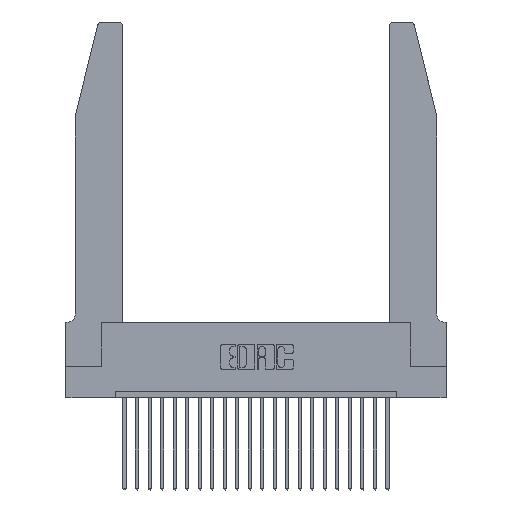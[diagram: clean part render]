
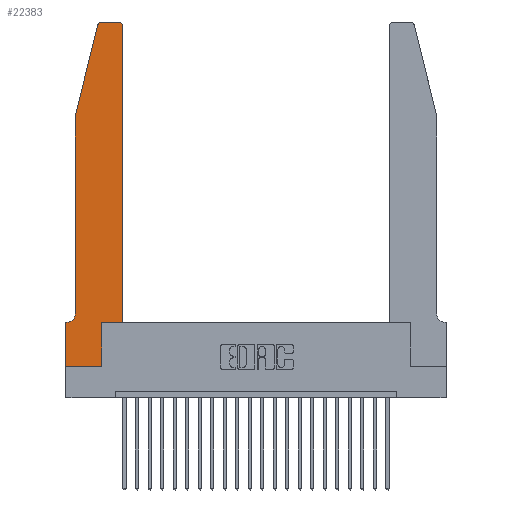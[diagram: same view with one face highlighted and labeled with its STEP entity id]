
A CAD part, top view. The second image highlights one B-rep face of the part: STEP entity #22383.
In plain terms, the highlighted planar face has unit normal (0, 0, 1).
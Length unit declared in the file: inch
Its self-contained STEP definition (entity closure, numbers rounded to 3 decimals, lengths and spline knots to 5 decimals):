
#57 = EDGE_CURVE ( 'NONE', #18648, #10782, #5771, .T. ) ;
#76 = DIRECTION ( 'NONE',  ( 0., 0., 1. ) ) ;
#520 = CARTESIAN_POINT ( 'NONE',  ( 0.0055, 0.35, 0.37 ) ) ;
#789 = VECTOR ( 'NONE', #22479, 39.37008 ) ;
#925 = VERTEX_POINT ( 'NONE', #14984 ) ;
#985 = CARTESIAN_POINT ( 'NONE',  ( 0., 0., 0.37 ) ) ;
#1343 = CARTESIAN_POINT ( 'NONE',  ( 0.25487, 2.72718, 0.37 ) ) ;
#1542 = DIRECTION ( 'NONE',  ( -1., 0., 0. ) ) ;
#2659 = VECTOR ( 'NONE', #9525, 39.37008 ) ;
#2760 = LINE ( 'NONE', #3527, #7111 ) ;
#2867 = VERTEX_POINT ( 'NONE', #16694 ) ;
#2967 = ORIENTED_EDGE ( 'NONE', *, *, #15690, .T. ) ;
#3189 = DIRECTION ( 'NONE',  ( 0., 0., 1. ) ) ;
#3259 = VECTOR ( 'NONE', #15316, 39.37008 ) ;
#3527 = CARTESIAN_POINT ( 'NONE',  ( 0.0755, 0.35, 0.37 ) ) ;
#3713 = VERTEX_POINT ( 'NONE', #18290 ) ;
#3759 = DIRECTION ( 'NONE',  ( -0.239, -0.971, 0. ) ) ;
#4540 = LINE ( 'NONE', #6917, #12961 ) ;
#4722 = CIRCLE ( 'NONE', #13330, 0.03 ) ;
#5266 = EDGE_CURVE ( 'NONE', #13035, #9064, #4540, .T. ) ;
#5589 = ORIENTED_EDGE ( 'NONE', *, *, #16961, .T. ) ;
#5689 = CARTESIAN_POINT ( 'NONE',  ( 0.0755, 2., 0.37 ) ) ;
#5757 = EDGE_CURVE ( 'NONE', #21542, #925, #2760, .T. ) ;
#5771 = LINE ( 'NONE', #13590, #789 ) ;
#6016 = VECTOR ( 'NONE', #3759, 39.37008 ) ;
#6346 = DIRECTION ( 'NONE',  ( 0., -1., 0. ) ) ;
#6392 = DIRECTION ( 'NONE',  ( 1., 0., 0. ) ) ;
#6635 = AXIS2_PLACEMENT_3D ( 'NONE', #16191, #10745, #7147 ) ;
#6715 = LINE ( 'NONE', #20277, #12856 ) ;
#6917 = CARTESIAN_POINT ( 'NONE',  ( 0.2605, 2.75, 0.37 ) ) ;
#6986 = EDGE_CURVE ( 'NONE', #9064, #9731, #4722, .T. ) ;
#7058 = EDGE_CURVE ( 'NONE', #19917, #3713, #15735, .T. ) ;
#7111 = VECTOR ( 'NONE', #1542, 39.37008 ) ;
#7147 = DIRECTION ( 'NONE',  ( -1., 0., 0. ) ) ;
#7605 = CARTESIAN_POINT ( 'NONE',  ( 0.2865, 0.35, 0.37 ) ) ;
#8390 = EDGE_LOOP ( 'NONE', ( #17396, #19748, #16897, #23469, #23577, #16543, #2967, #21806, #5589, #14961, #10084, #13837 ) ) ;
#8466 = CARTESIAN_POINT ( 'NONE',  ( 0., 0., 0.37 ) ) ;
#8567 = CIRCLE ( 'NONE', #9382, 0.03 ) ;
#8801 = DIRECTION ( 'NONE',  ( -1., 0., 0. ) ) ;
#9064 = VERTEX_POINT ( 'NONE', #21634 ) ;
#9091 = DIRECTION ( 'NONE',  ( 1., 0., 0. ) ) ;
#9142 = VECTOR ( 'NONE', #6346, 39.37008 ) ;
#9382 = AXIS2_PLACEMENT_3D ( 'NONE', #16250, #3189, #16169 ) ;
#9525 = DIRECTION ( 'NONE',  ( 0., -1., 0. ) ) ;
#9731 = VERTEX_POINT ( 'NONE', #1343 ) ;
#9945 = CARTESIAN_POINT ( 'NONE',  ( 0.4205, 2.75, 0.37 ) ) ;
#10084 = ORIENTED_EDGE ( 'NONE', *, *, #18473, .T. ) ;
#10219 = CARTESIAN_POINT ( 'NONE',  ( 0.4505, 0.35, 0.37 ) ) ;
#10232 = CARTESIAN_POINT ( 'NONE',  ( 0., 0.35, 0.37 ) ) ;
#10745 = DIRECTION ( 'NONE',  ( 0., 0., -1. ) ) ;
#10782 = VERTEX_POINT ( 'NONE', #22024 ) ;
#11005 = LINE ( 'NONE', #18827, #13887 ) ;
#11461 = VERTEX_POINT ( 'NONE', #10219 ) ;
#11842 = LINE ( 'NONE', #21799, #6016 ) ;
#12260 = EDGE_CURVE ( 'NONE', #9731, #19917, #11842, .T. ) ;
#12856 = VECTOR ( 'NONE', #9091, 39.37008 ) ;
#12961 = VECTOR ( 'NONE', #8801, 39.37008 ) ;
#13035 = VERTEX_POINT ( 'NONE', #9945 ) ;
#13330 = AXIS2_PLACEMENT_3D ( 'NONE', #22915, #76, #18743 ) ;
#13590 = CARTESIAN_POINT ( 'NONE',  ( 0., 0., 0.37 ) ) ;
#13837 = ORIENTED_EDGE ( 'NONE', *, *, #15047, .T. ) ;
#13887 = VECTOR ( 'NONE', #17045, 39.37008 ) ;
#13909 = CIRCLE ( 'NONE', #6635, 0.07 ) ;
#14961 = ORIENTED_EDGE ( 'NONE', *, *, #22709, .T. ) ;
#14984 = CARTESIAN_POINT ( 'NONE',  ( 0., 0.35, 0.37 ) ) ;
#15047 = EDGE_CURVE ( 'NONE', #17881, #13035, #8567, .T. ) ;
#15316 = DIRECTION ( 'NONE',  ( 0., 1., 0. ) ) ;
#15471 = FACE_OUTER_BOUND ( 'NONE', #8390, .T. ) ;
#15690 = EDGE_CURVE ( 'NONE', #925, #18648, #17239, .T. ) ;
#15735 = LINE ( 'NONE', #5689, #2659 ) ;
#15915 = PLANE ( 'NONE',  #17508 ) ;
#16169 = DIRECTION ( 'NONE',  ( 1., 0., 0. ) ) ;
#16191 = CARTESIAN_POINT ( 'NONE',  ( 0.0055, 0.42, 0.37 ) ) ;
#16250 = CARTESIAN_POINT ( 'NONE',  ( 0.4205, 2.72, 0.37 ) ) ;
#16543 = ORIENTED_EDGE ( 'NONE', *, *, #5757, .T. ) ;
#16694 = CARTESIAN_POINT ( 'NONE',  ( 0.2865, 0.35, 0.37 ) ) ;
#16897 = ORIENTED_EDGE ( 'NONE', *, *, #12260, .T. ) ;
#16961 = EDGE_CURVE ( 'NONE', #10782, #2867, #22086, .T. ) ;
#17045 = DIRECTION ( 'NONE',  ( 0., 1., 0. ) ) ;
#17239 = LINE ( 'NONE', #8466, #9142 ) ;
#17396 = ORIENTED_EDGE ( 'NONE', *, *, #5266, .T. ) ;
#17508 = AXIS2_PLACEMENT_3D ( 'NONE', #10232, #21212, #6392 ) ;
#17794 = EDGE_CURVE ( 'NONE', #3713, #21542, #13909, .T. ) ;
#17881 = VERTEX_POINT ( 'NONE', #20757 ) ;
#18290 = CARTESIAN_POINT ( 'NONE',  ( 0.0755, 0.42, 0.37 ) ) ;
#18473 = EDGE_CURVE ( 'NONE', #11461, #17881, #11005, .T. ) ;
#18648 = VERTEX_POINT ( 'NONE', #985 ) ;
#18743 = DIRECTION ( 'NONE',  ( 1., 0., 0. ) ) ;
#18827 = CARTESIAN_POINT ( 'NONE',  ( 0.4505, 0.35, 0.37 ) ) ;
#19748 = ORIENTED_EDGE ( 'NONE', *, *, #6986, .T. ) ;
#19917 = VERTEX_POINT ( 'NONE', #20521 ) ;
#20277 = CARTESIAN_POINT ( 'NONE',  ( 0.4505, 0.35, 0.37 ) ) ;
#20521 = CARTESIAN_POINT ( 'NONE',  ( 0.0755, 2., 0.37 ) ) ;
#20757 = CARTESIAN_POINT ( 'NONE',  ( 0.4505, 2.72, 0.37 ) ) ;
#21212 = DIRECTION ( 'NONE',  ( 0., 0., 1. ) ) ;
#21542 = VERTEX_POINT ( 'NONE', #520 ) ;
#21634 = CARTESIAN_POINT ( 'NONE',  ( 0.284, 2.75, 0.37 ) ) ;
#21799 = CARTESIAN_POINT ( 'NONE',  ( 0.0755, 2., 0.37 ) ) ;
#21806 = ORIENTED_EDGE ( 'NONE', *, *, #57, .T. ) ;
#22024 = CARTESIAN_POINT ( 'NONE',  ( 0.2865, 0., 0.37 ) ) ;
#22086 = LINE ( 'NONE', #7605, #3259 ) ;
#22383 = ADVANCED_FACE ( 'NONE', ( #15471 ), #15915, .T. ) ;
#22479 = DIRECTION ( 'NONE',  ( 1., 0., 0. ) ) ;
#22709 = EDGE_CURVE ( 'NONE', #2867, #11461, #6715, .T. ) ;
#22915 = CARTESIAN_POINT ( 'NONE',  ( 0.284, 2.72, 0.37 ) ) ;
#23469 = ORIENTED_EDGE ( 'NONE', *, *, #7058, .T. ) ;
#23577 = ORIENTED_EDGE ( 'NONE', *, *, #17794, .T. ) ;
